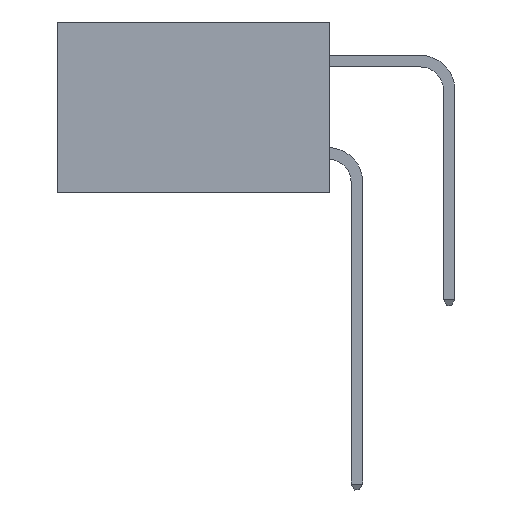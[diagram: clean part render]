
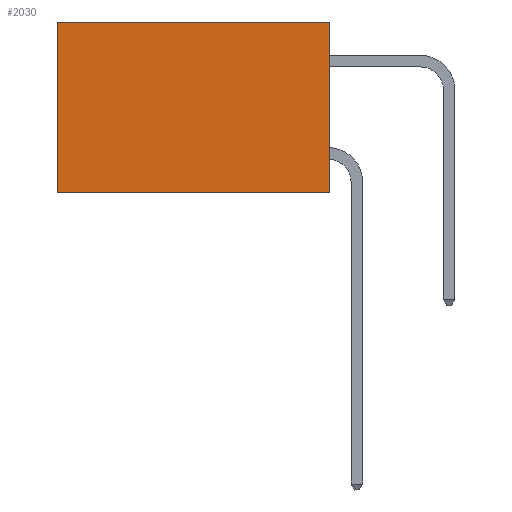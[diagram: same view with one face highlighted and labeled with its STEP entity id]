
A CAD part, left-side view. The second image highlights one B-rep face of the part: STEP entity #2030.
In plain terms, the highlighted planar face has unit normal (-1, 0, 0).
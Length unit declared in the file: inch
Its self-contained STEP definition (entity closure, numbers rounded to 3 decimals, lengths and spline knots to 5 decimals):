
#16 = DIRECTION ( 'NONE',  ( 0., 0., -1. ) ) ;
#44 = VERTEX_POINT ( 'NONE', #9498 ) ;
#328 = LINE ( 'NONE', #9547, #2731 ) ;
#458 = VERTEX_POINT ( 'NONE', #10373 ) ;
#654 = ORIENTED_EDGE ( 'NONE', *, *, #6891, .T. ) ;
#1113 = VERTEX_POINT ( 'NONE', #3459 ) ;
#1202 = AXIS2_PLACEMENT_3D ( 'NONE', #6711, #6529, #6518 ) ;
#1223 = VECTOR ( 'NONE', #2194, 39.37008 ) ;
#1624 = FACE_OUTER_BOUND ( 'NONE', #5115, .T. ) ;
#1980 = CARTESIAN_POINT ( 'NONE',  ( 0.277, 0., -0.37 ) ) ;
#2030 = ADVANCED_FACE ( 'NONE', ( #1624 ), #6573, .F. ) ;
#2194 = DIRECTION ( 'NONE',  ( 0., 1., 0. ) ) ;
#2218 = CARTESIAN_POINT ( 'NONE',  ( 0.277, 0., 0. ) ) ;
#2413 = EDGE_CURVE ( 'NONE', #1113, #2720, #9200, .T. ) ;
#2558 = EDGE_CURVE ( 'NONE', #458, #44, #8402, .T. ) ;
#2635 = EDGE_CURVE ( 'NONE', #1113, #458, #3648, .T. ) ;
#2720 = VERTEX_POINT ( 'NONE', #6168 ) ;
#2731 = VECTOR ( 'NONE', #4291, 39.37008 ) ;
#3428 = VECTOR ( 'NONE', #16, 39.37008 ) ;
#3459 = CARTESIAN_POINT ( 'NONE',  ( 0.277, 0., 0. ) ) ;
#3495 = ORIENTED_EDGE ( 'NONE', *, *, #2413, .T. ) ;
#3589 = CARTESIAN_POINT ( 'NONE',  ( 0.277, 0., -0.37 ) ) ;
#3648 = LINE ( 'NONE', #1980, #3428 ) ;
#4291 = DIRECTION ( 'NONE',  ( 0., 0., -1. ) ) ;
#5115 = EDGE_LOOP ( 'NONE', ( #654, #7301, #9266, #3495 ) ) ;
#6168 = CARTESIAN_POINT ( 'NONE',  ( 0.277, 0.59, 0. ) ) ;
#6518 = DIRECTION ( 'NONE',  ( 0., 0., -1. ) ) ;
#6529 = DIRECTION ( 'NONE',  ( 1., 0., 0. ) ) ;
#6573 = PLANE ( 'NONE',  #1202 ) ;
#6666 = VECTOR ( 'NONE', #8866, 39.37008 ) ;
#6711 = CARTESIAN_POINT ( 'NONE',  ( 0.277, 0., -0.37 ) ) ;
#6891 = EDGE_CURVE ( 'NONE', #2720, #44, #328, .T. ) ;
#7301 = ORIENTED_EDGE ( 'NONE', *, *, #2558, .F. ) ;
#8402 = LINE ( 'NONE', #3589, #6666 ) ;
#8866 = DIRECTION ( 'NONE',  ( 0., 1., 0. ) ) ;
#9200 = LINE ( 'NONE', #2218, #1223 ) ;
#9266 = ORIENTED_EDGE ( 'NONE', *, *, #2635, .F. ) ;
#9498 = CARTESIAN_POINT ( 'NONE',  ( 0.277, 0.59, -0.37 ) ) ;
#9547 = CARTESIAN_POINT ( 'NONE',  ( 0.277, 0.59, -0.37 ) ) ;
#10373 = CARTESIAN_POINT ( 'NONE',  ( 0.277, 0., -0.37 ) ) ;
